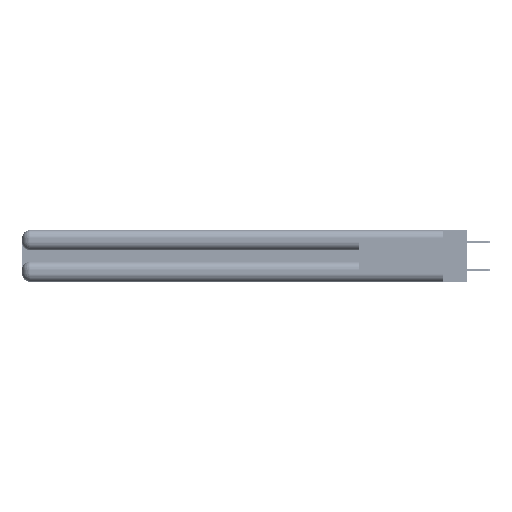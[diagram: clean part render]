
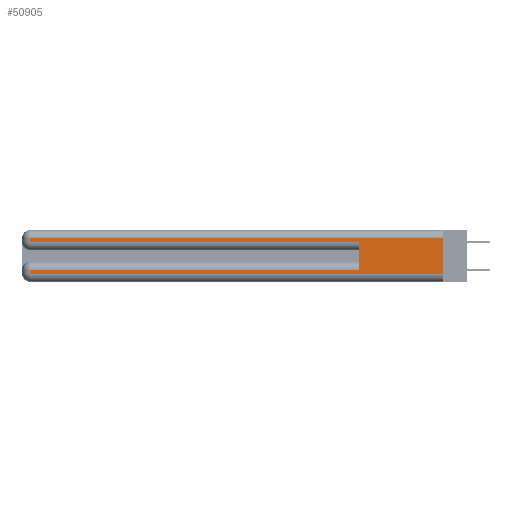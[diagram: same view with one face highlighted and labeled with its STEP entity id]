
A CAD part, left-side view. The second image highlights one B-rep face of the part: STEP entity #50905.
In plain terms, the highlighted planar face has unit normal (-1, 0, 0).
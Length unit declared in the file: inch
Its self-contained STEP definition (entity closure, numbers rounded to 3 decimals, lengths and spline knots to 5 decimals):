
#283 = LINE ( 'NONE', #54310, #34819 ) ;
#1412 = ORIENTED_EDGE ( 'NONE', *, *, #28649, .F. ) ;
#2027 = VECTOR ( 'NONE', #27112, 39.37008 ) ;
#2402 = EDGE_CURVE ( 'NONE', #36367, #19228, #14020, .T. ) ;
#2783 = CARTESIAN_POINT ( 'NONE',  ( 0., 2.94, 0.31 ) ) ;
#3620 = EDGE_CURVE ( 'NONE', #24332, #39183, #14603, .T. ) ;
#5292 = ORIENTED_EDGE ( 'NONE', *, *, #3620, .T. ) ;
#5630 = DIRECTION ( 'NONE',  ( 0., 0., -1. ) ) ;
#6046 = ORIENTED_EDGE ( 'NONE', *, *, #49761, .T. ) ;
#7147 = DIRECTION ( 'NONE',  ( 0., 1., 0. ) ) ;
#9128 = VERTEX_POINT ( 'NONE', #54833 ) ;
#9995 = ORIENTED_EDGE ( 'NONE', *, *, #23412, .T. ) ;
#10009 = ORIENTED_EDGE ( 'NONE', *, *, #27649, .T. ) ;
#11052 = DIRECTION ( 'NONE',  ( 0., 0., -1. ) ) ;
#13393 = CARTESIAN_POINT ( 'NONE',  ( 0., 0., 0.085 ) ) ;
#14020 = LINE ( 'NONE', #31601, #2027 ) ;
#14603 = LINE ( 'NONE', #16752, #46097 ) ;
#15481 = CARTESIAN_POINT ( 'NONE',  ( 0., 0., 0.285 ) ) ;
#15544 = VECTOR ( 'NONE', #20022, 39.37008 ) ;
#16752 = CARTESIAN_POINT ( 'NONE',  ( 0., 2.94, 0.37 ) ) ;
#19228 = VERTEX_POINT ( 'NONE', #38592 ) ;
#20022 = DIRECTION ( 'NONE',  ( 0., -1., 0. ) ) ;
#20614 = LINE ( 'NONE', #13393, #57465 ) ;
#23412 = EDGE_CURVE ( 'NONE', #39183, #50235, #283, .T. ) ;
#23478 = VECTOR ( 'NONE', #11052, 39.37008 ) ;
#23686 = LINE ( 'NONE', #34147, #35609 ) ;
#23788 = CARTESIAN_POINT ( 'NONE',  ( 0., 2.94, 0.285 ) ) ;
#24332 = VERTEX_POINT ( 'NONE', #55908 ) ;
#24869 = CARTESIAN_POINT ( 'NONE',  ( 0., 2.94, 0.06 ) ) ;
#26288 = LINE ( 'NONE', #33538, #23478 ) ;
#26443 = CARTESIAN_POINT ( 'NONE',  ( 0., 0., 0.37 ) ) ;
#26546 = LINE ( 'NONE', #26443, #39869 ) ;
#27112 = DIRECTION ( 'NONE',  ( 0., 0., 1. ) ) ;
#27649 = EDGE_CURVE ( 'NONE', #36367, #24332, #20614, .T. ) ;
#27705 = DIRECTION ( 'NONE',  ( 0., -1., 0. ) ) ;
#28174 = EDGE_LOOP ( 'NONE', ( #1412, #45918, #6046, #43477, #31133, #10009, #5292, #9995 ) ) ;
#28649 = EDGE_CURVE ( 'NONE', #9128, #50235, #26546, .T. ) ;
#31133 = ORIENTED_EDGE ( 'NONE', *, *, #2402, .F. ) ;
#31601 = CARTESIAN_POINT ( 'NONE',  ( 0., 0.6, 0.145 ) ) ;
#33292 = EDGE_CURVE ( 'NONE', #9128, #55808, #23686, .T. ) ;
#33538 = CARTESIAN_POINT ( 'NONE',  ( 0., 2.94, 0.37 ) ) ;
#34147 = CARTESIAN_POINT ( 'NONE',  ( 0., 0., 0.31 ) ) ;
#34819 = VECTOR ( 'NONE', #27705, 39.37008 ) ;
#35609 = VECTOR ( 'NONE', #7147, 39.37008 ) ;
#36367 = VERTEX_POINT ( 'NONE', #39724 ) ;
#38592 = CARTESIAN_POINT ( 'NONE',  ( 0., 0.6, 0.285 ) ) ;
#39131 = DIRECTION ( 'NONE',  ( 0., 0., -1. ) ) ;
#39183 = VERTEX_POINT ( 'NONE', #24869 ) ;
#39432 = LINE ( 'NONE', #15481, #15544 ) ;
#39724 = CARTESIAN_POINT ( 'NONE',  ( 0., 0.6, 0.085 ) ) ;
#39869 = VECTOR ( 'NONE', #57452, 39.37008 ) ;
#41256 = CARTESIAN_POINT ( 'NONE',  ( 0., 0., 0.06 ) ) ;
#41370 = DIRECTION ( 'NONE',  ( 1., 0., 0. ) ) ;
#42981 = AXIS2_PLACEMENT_3D ( 'NONE', #45811, #41370, #5630 ) ;
#43477 = ORIENTED_EDGE ( 'NONE', *, *, #51044, .T. ) ;
#44371 = DIRECTION ( 'NONE',  ( 0., 1., 0. ) ) ;
#45811 = CARTESIAN_POINT ( 'NONE',  ( 0., 0., 0.37 ) ) ;
#45918 = ORIENTED_EDGE ( 'NONE', *, *, #33292, .T. ) ;
#46097 = VECTOR ( 'NONE', #39131, 39.37008 ) ;
#46333 = FACE_OUTER_BOUND ( 'NONE', #28174, .T. ) ;
#49761 = EDGE_CURVE ( 'NONE', #55808, #50923, #26288, .T. ) ;
#50235 = VERTEX_POINT ( 'NONE', #41256 ) ;
#50905 = ADVANCED_FACE ( 'NONE', ( #46333 ), #54691, .F. ) ;
#50923 = VERTEX_POINT ( 'NONE', #23788 ) ;
#51044 = EDGE_CURVE ( 'NONE', #50923, #19228, #39432, .T. ) ;
#54310 = CARTESIAN_POINT ( 'NONE',  ( 0., 0., 0.06 ) ) ;
#54691 = PLANE ( 'NONE',  #42981 ) ;
#54833 = CARTESIAN_POINT ( 'NONE',  ( 0., 0., 0.31 ) ) ;
#55808 = VERTEX_POINT ( 'NONE', #2783 ) ;
#55908 = CARTESIAN_POINT ( 'NONE',  ( 0., 2.94, 0.085 ) ) ;
#57452 = DIRECTION ( 'NONE',  ( 0., 0., -1. ) ) ;
#57465 = VECTOR ( 'NONE', #44371, 39.37008 ) ;
